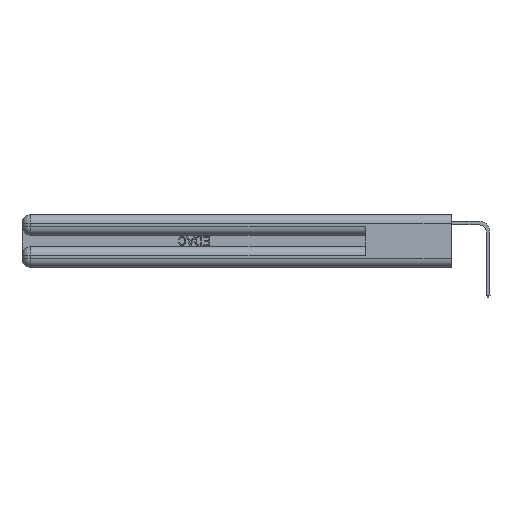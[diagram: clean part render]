
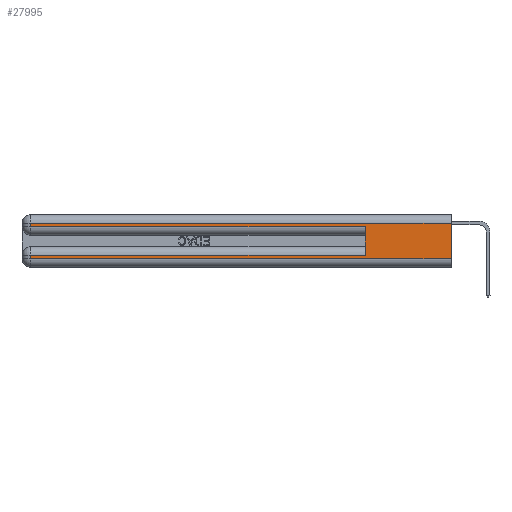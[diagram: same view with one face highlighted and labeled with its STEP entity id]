
A CAD part, left-side view. The second image highlights one B-rep face of the part: STEP entity #27995.
In plain terms, the highlighted planar face has unit normal (-1, 0, 0).
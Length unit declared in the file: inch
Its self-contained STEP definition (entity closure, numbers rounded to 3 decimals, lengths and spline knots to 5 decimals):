
#30 = EDGE_CURVE ( 'NONE', #8783, #1232, #26310, .T. ) ;
#34 = DIRECTION ( 'NONE',  ( 1., 0., 0. ) ) ;
#960 = LINE ( 'NONE', #19022, #14874 ) ;
#1232 = VERTEX_POINT ( 'NONE', #22933 ) ;
#1245 = EDGE_CURVE ( 'NONE', #12645, #13547, #960, .T. ) ;
#2545 = DIRECTION ( 'NONE',  ( 0., 0., 1. ) ) ;
#2777 = EDGE_CURVE ( 'NONE', #11032, #12645, #26615, .T. ) ;
#2928 = EDGE_CURVE ( 'NONE', #14901, #1232, #5934, .T. ) ;
#2986 = CARTESIAN_POINT ( 'NONE',  ( 0., 2.94, 0.06 ) ) ;
#3601 = CARTESIAN_POINT ( 'NONE',  ( 0., 0., 0.31 ) ) ;
#3774 = CARTESIAN_POINT ( 'NONE',  ( 0., 0.6, 0.285 ) ) ;
#4003 = CARTESIAN_POINT ( 'NONE',  ( 0., 0., 0.31 ) ) ;
#4133 = LINE ( 'NONE', #16827, #16189 ) ;
#4622 = CARTESIAN_POINT ( 'NONE',  ( 0., 0., 0.37 ) ) ;
#4722 = ORIENTED_EDGE ( 'NONE', *, *, #9915, .T. ) ;
#4779 = PLANE ( 'NONE',  #27535 ) ;
#5387 = ORIENTED_EDGE ( 'NONE', *, *, #19285, .T. ) ;
#5934 = LINE ( 'NONE', #12361, #27925 ) ;
#5989 = DIRECTION ( 'NONE',  ( 0., 0., -1. ) ) ;
#6817 = CARTESIAN_POINT ( 'NONE',  ( 0., 0.6, 0.145 ) ) ;
#7511 = EDGE_CURVE ( 'NONE', #20324, #13547, #13408, .T. ) ;
#7629 = DIRECTION ( 'NONE',  ( 0., -1., 0. ) ) ;
#7750 = CARTESIAN_POINT ( 'NONE',  ( 0., 0., 0.085 ) ) ;
#7775 = ORIENTED_EDGE ( 'NONE', *, *, #19286, .T. ) ;
#8783 = VERTEX_POINT ( 'NONE', #3601 ) ;
#8999 = ORIENTED_EDGE ( 'NONE', *, *, #7511, .F. ) ;
#9884 = LINE ( 'NONE', #7750, #12824 ) ;
#9915 = EDGE_CURVE ( 'NONE', #20324, #17095, #9884, .T. ) ;
#11032 = VERTEX_POINT ( 'NONE', #27947 ) ;
#11294 = ORIENTED_EDGE ( 'NONE', *, *, #2777, .T. ) ;
#11333 = ORIENTED_EDGE ( 'NONE', *, *, #30, .F. ) ;
#11352 = CARTESIAN_POINT ( 'NONE',  ( 0., 2.94, 0.085 ) ) ;
#11413 = EDGE_LOOP ( 'NONE', ( #11333, #5387, #11294, #24600, #8999, #4722, #7775, #25124 ) ) ;
#11798 = CARTESIAN_POINT ( 'NONE',  ( 0., 2.94, 0.37 ) ) ;
#12361 = CARTESIAN_POINT ( 'NONE',  ( 0., 0., 0.06 ) ) ;
#12645 = VERTEX_POINT ( 'NONE', #27373 ) ;
#12730 = VECTOR ( 'NONE', #17787, 39.37008 ) ;
#12824 = VECTOR ( 'NONE', #13754, 39.37008 ) ;
#13408 = LINE ( 'NONE', #6817, #23463 ) ;
#13547 = VERTEX_POINT ( 'NONE', #3774 ) ;
#13754 = DIRECTION ( 'NONE',  ( 0., 1., 0. ) ) ;
#14874 = VECTOR ( 'NONE', #18418, 39.37008 ) ;
#14901 = VERTEX_POINT ( 'NONE', #2986 ) ;
#16189 = VECTOR ( 'NONE', #5989, 39.37008 ) ;
#16827 = CARTESIAN_POINT ( 'NONE',  ( 0., 2.94, 0.37 ) ) ;
#17095 = VERTEX_POINT ( 'NONE', #11352 ) ;
#17211 = DIRECTION ( 'NONE',  ( 0., 0., -1. ) ) ;
#17481 = CARTESIAN_POINT ( 'NONE',  ( 0., 0.6, 0.085 ) ) ;
#17544 = VECTOR ( 'NONE', #26089, 39.37008 ) ;
#17787 = DIRECTION ( 'NONE',  ( 0., 0., -1. ) ) ;
#18418 = DIRECTION ( 'NONE',  ( 0., -1., 0. ) ) ;
#19022 = CARTESIAN_POINT ( 'NONE',  ( 0., 0., 0.285 ) ) ;
#19285 = EDGE_CURVE ( 'NONE', #8783, #11032, #23768, .T. ) ;
#19286 = EDGE_CURVE ( 'NONE', #17095, #14901, #4133, .T. ) ;
#19553 = FACE_OUTER_BOUND ( 'NONE', #11413, .T. ) ;
#19911 = VECTOR ( 'NONE', #17211, 39.37008 ) ;
#20324 = VERTEX_POINT ( 'NONE', #17481 ) ;
#22933 = CARTESIAN_POINT ( 'NONE',  ( 0., 0., 0.06 ) ) ;
#23463 = VECTOR ( 'NONE', #2545, 39.37008 ) ;
#23768 = LINE ( 'NONE', #4003, #17544 ) ;
#24168 = DIRECTION ( 'NONE',  ( 0., 0., -1. ) ) ;
#24600 = ORIENTED_EDGE ( 'NONE', *, *, #1245, .T. ) ;
#25124 = ORIENTED_EDGE ( 'NONE', *, *, #2928, .T. ) ;
#26089 = DIRECTION ( 'NONE',  ( 0., 1., 0. ) ) ;
#26310 = LINE ( 'NONE', #4622, #19911 ) ;
#26615 = LINE ( 'NONE', #11798, #12730 ) ;
#27373 = CARTESIAN_POINT ( 'NONE',  ( 0., 2.94, 0.285 ) ) ;
#27535 = AXIS2_PLACEMENT_3D ( 'NONE', #28322, #34, #24168 ) ;
#27925 = VECTOR ( 'NONE', #7629, 39.37008 ) ;
#27947 = CARTESIAN_POINT ( 'NONE',  ( 0., 2.94, 0.31 ) ) ;
#27995 = ADVANCED_FACE ( 'NONE', ( #19553 ), #4779, .F. ) ;
#28322 = CARTESIAN_POINT ( 'NONE',  ( 0., 0., 0.37 ) ) ;
